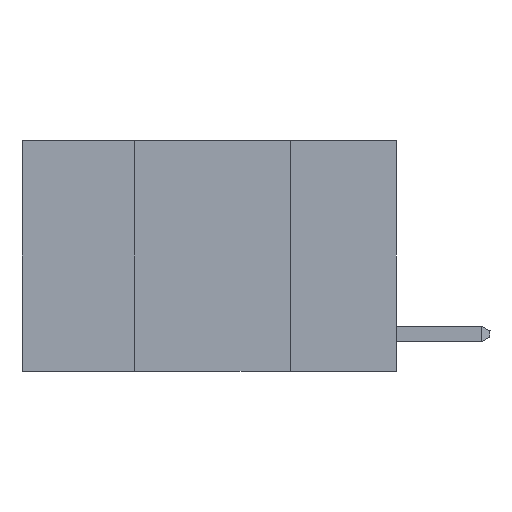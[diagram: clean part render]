
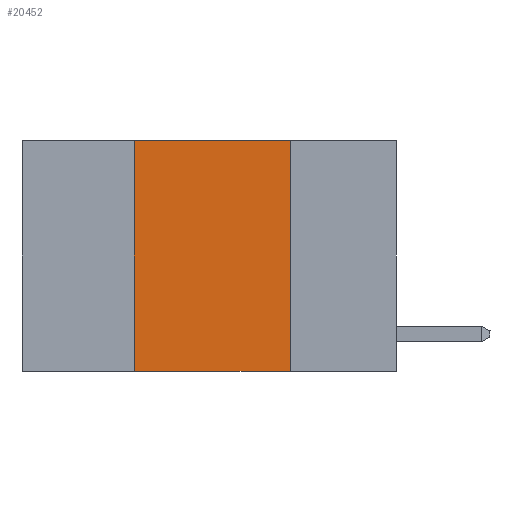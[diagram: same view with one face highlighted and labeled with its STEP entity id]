
A CAD part, left-side view. The second image highlights one B-rep face of the part: STEP entity #20452.
In plain terms, the highlighted planar face has unit normal (-1, 0, 0).
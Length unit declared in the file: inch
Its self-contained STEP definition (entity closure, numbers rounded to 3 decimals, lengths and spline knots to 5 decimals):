
#1733 = ORIENTED_EDGE ( 'NONE', *, *, #17032, .F. ) ;
#2860 = LINE ( 'NONE', #18365, #19492 ) ;
#4649 = AXIS2_PLACEMENT_3D ( 'NONE', #14921, #22982, #10945 ) ;
#5675 = VECTOR ( 'NONE', #24570, 39.37008 ) ;
#5795 = ORIENTED_EDGE ( 'NONE', *, *, #12978, .F. ) ;
#6313 = DIRECTION ( 'NONE',  ( 0., -1., 0. ) ) ;
#6603 = CARTESIAN_POINT ( 'NONE',  ( 0., 0.6, 0. ) ) ;
#8638 = CARTESIAN_POINT ( 'NONE',  ( 0., 0.17, -0.37 ) ) ;
#8954 = EDGE_LOOP ( 'NONE', ( #5795, #22429, #1733, #12391 ) ) ;
#10174 = CARTESIAN_POINT ( 'NONE',  ( 0., 0.17, 0. ) ) ;
#10476 = VERTEX_POINT ( 'NONE', #21772 ) ;
#10945 = DIRECTION ( 'NONE',  ( 0., 0., -1. ) ) ;
#11176 = FACE_OUTER_BOUND ( 'NONE', #8954, .T. ) ;
#11196 = CARTESIAN_POINT ( 'NONE',  ( 0., 0.42, 0. ) ) ;
#12214 = DIRECTION ( 'NONE',  ( 0., 0., -1. ) ) ;
#12391 = ORIENTED_EDGE ( 'NONE', *, *, #18376, .T. ) ;
#12978 = EDGE_CURVE ( 'NONE', #19888, #25868, #14776, .T. ) ;
#13139 = EDGE_CURVE ( 'NONE', #22156, #19888, #16331, .T. ) ;
#13145 = CARTESIAN_POINT ( 'NONE',  ( 0., 0.42, 0. ) ) ;
#14776 = LINE ( 'NONE', #10174, #20131 ) ;
#14820 = LINE ( 'NONE', #13145, #25463 ) ;
#14921 = CARTESIAN_POINT ( 'NONE',  ( 0., 0.6, 0. ) ) ;
#16331 = LINE ( 'NONE', #6603, #5675 ) ;
#17032 = EDGE_CURVE ( 'NONE', #10476, #22156, #14820, .T. ) ;
#17255 = CARTESIAN_POINT ( 'NONE',  ( 0., 0.17, 0. ) ) ;
#18365 = CARTESIAN_POINT ( 'NONE',  ( 0., 0.6, -0.37 ) ) ;
#18376 = EDGE_CURVE ( 'NONE', #10476, #25868, #2860, .T. ) ;
#19143 = DIRECTION ( 'NONE',  ( 0., 0., 1. ) ) ;
#19492 = VECTOR ( 'NONE', #6313, 39.37008 ) ;
#19888 = VERTEX_POINT ( 'NONE', #17255 ) ;
#20131 = VECTOR ( 'NONE', #12214, 39.37008 ) ;
#20452 = ADVANCED_FACE ( 'NONE', ( #11176 ), #20989, .F. ) ;
#20989 = PLANE ( 'NONE',  #4649 ) ;
#21772 = CARTESIAN_POINT ( 'NONE',  ( 0., 0.42, -0.37 ) ) ;
#22156 = VERTEX_POINT ( 'NONE', #11196 ) ;
#22429 = ORIENTED_EDGE ( 'NONE', *, *, #13139, .F. ) ;
#22982 = DIRECTION ( 'NONE',  ( 1., 0., 0. ) ) ;
#24570 = DIRECTION ( 'NONE',  ( 0., -1., 0. ) ) ;
#25463 = VECTOR ( 'NONE', #19143, 39.37008 ) ;
#25868 = VERTEX_POINT ( 'NONE', #8638 ) ;
